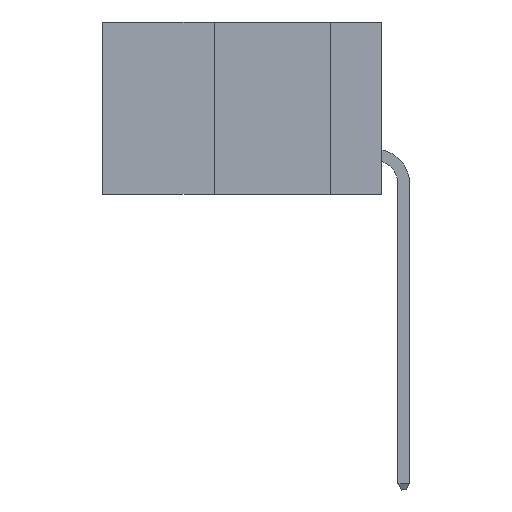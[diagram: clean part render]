
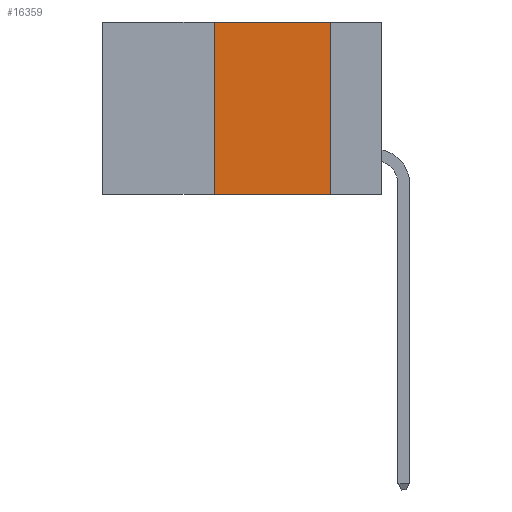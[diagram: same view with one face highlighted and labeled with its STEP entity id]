
A CAD part, left-side view. The second image highlights one B-rep face of the part: STEP entity #16359.
In plain terms, the highlighted planar face has unit normal (-1, 0, 0).
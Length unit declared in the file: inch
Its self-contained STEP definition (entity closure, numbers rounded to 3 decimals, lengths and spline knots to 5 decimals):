
#988 = CARTESIAN_POINT ( 'NONE',  ( 0., 0.11, -0.37 ) ) ;
#1011 = CARTESIAN_POINT ( 'NONE',  ( 0., 0.6, -0.37 ) ) ;
#2182 = ORIENTED_EDGE ( 'NONE', *, *, #25125, .F. ) ;
#2275 = DIRECTION ( 'NONE',  ( 0., 0., -1. ) ) ;
#2848 = EDGE_LOOP ( 'NONE', ( #23117, #32488, #2182, #19437 ) ) ;
#2861 = CARTESIAN_POINT ( 'NONE',  ( 0., 0.36, -0.37 ) ) ;
#3263 = VECTOR ( 'NONE', #2275, 39.37008 ) ;
#3646 = DIRECTION ( 'NONE',  ( 0., 0., 1. ) ) ;
#4651 = CARTESIAN_POINT ( 'NONE',  ( 0., 0.36, 0. ) ) ;
#7164 = EDGE_CURVE ( 'NONE', #27790, #28711, #37775, .T. ) ;
#7998 = CARTESIAN_POINT ( 'NONE',  ( 0., 0.6, 0. ) ) ;
#9132 = EDGE_CURVE ( 'NONE', #38164, #9626, #31573, .T. ) ;
#9439 = FACE_OUTER_BOUND ( 'NONE', #2848, .T. ) ;
#9626 = VERTEX_POINT ( 'NONE', #988 ) ;
#10024 = VECTOR ( 'NONE', #38560, 39.37008 ) ;
#16359 = ADVANCED_FACE ( 'NONE', ( #9439 ), #37435, .F. ) ;
#16716 = VECTOR ( 'NONE', #16956, 39.37008 ) ;
#16956 = DIRECTION ( 'NONE',  ( 0., -1., 0. ) ) ;
#19173 = CARTESIAN_POINT ( 'NONE',  ( 0., 0.36, 0. ) ) ;
#19437 = ORIENTED_EDGE ( 'NONE', *, *, #9132, .T. ) ;
#19718 = DIRECTION ( 'NONE',  ( 1., 0., 0. ) ) ;
#23117 = ORIENTED_EDGE ( 'NONE', *, *, #28716, .F. ) ;
#24371 = CARTESIAN_POINT ( 'NONE',  ( 0., 0.11, 0. ) ) ;
#25125 = EDGE_CURVE ( 'NONE', #38164, #27790, #30538, .T. ) ;
#27124 = VECTOR ( 'NONE', #3646, 39.37008 ) ;
#27746 = LINE ( 'NONE', #24371, #3263 ) ;
#27790 = VERTEX_POINT ( 'NONE', #4651 ) ;
#28673 = CARTESIAN_POINT ( 'NONE',  ( 0., 0.6, 0. ) ) ;
#28711 = VERTEX_POINT ( 'NONE', #39960 ) ;
#28716 = EDGE_CURVE ( 'NONE', #28711, #9626, #27746, .T. ) ;
#29839 = AXIS2_PLACEMENT_3D ( 'NONE', #28673, #19718, #38593 ) ;
#30538 = LINE ( 'NONE', #19173, #27124 ) ;
#31573 = LINE ( 'NONE', #1011, #10024 ) ;
#32488 = ORIENTED_EDGE ( 'NONE', *, *, #7164, .F. ) ;
#37435 = PLANE ( 'NONE',  #29839 ) ;
#37775 = LINE ( 'NONE', #7998, #16716 ) ;
#38164 = VERTEX_POINT ( 'NONE', #2861 ) ;
#38560 = DIRECTION ( 'NONE',  ( 0., -1., 0. ) ) ;
#38593 = DIRECTION ( 'NONE',  ( 0., 0., -1. ) ) ;
#39960 = CARTESIAN_POINT ( 'NONE',  ( 0., 0.11, 0. ) ) ;
